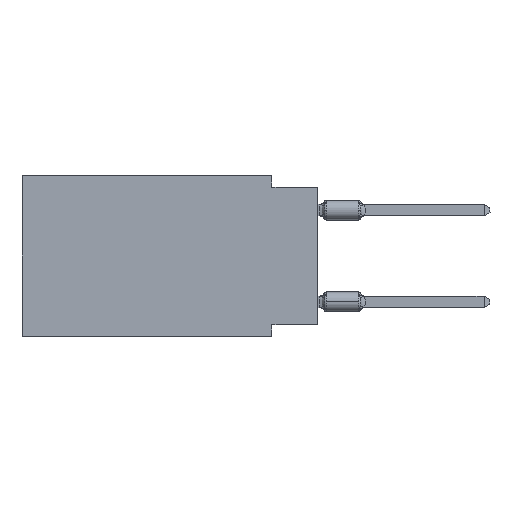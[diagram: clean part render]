
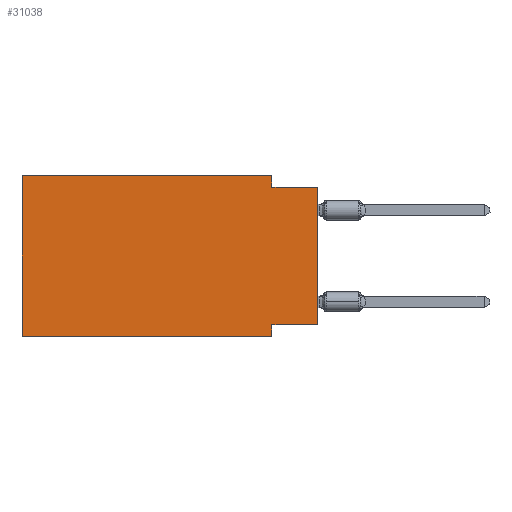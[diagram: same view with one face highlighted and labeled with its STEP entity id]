
A CAD part, left-side view. The second image highlights one B-rep face of the part: STEP entity #31038.
In plain terms, the highlighted planar face has unit normal (-1, 0, 0).
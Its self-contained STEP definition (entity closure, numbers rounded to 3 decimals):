
#113 = DIRECTION ( 'NONE',  ( 0., -1., 0. ) ) ;
#422 = VERTEX_POINT ( 'NONE', #11493 ) ;
#509 = DIRECTION ( 'NONE',  ( 0., 0., 1. ) ) ;
#956 = EDGE_CURVE ( 'NONE', #2455, #422, #2390, .T. ) ;
#1408 = EDGE_CURVE ( 'NONE', #10008, #23728, #19799, .T. ) ;
#2032 = VECTOR ( 'NONE', #21883, 1000. ) ;
#2119 = LINE ( 'NONE', #31627, #17342 ) ;
#2390 = LINE ( 'NONE', #9981, #16256 ) ;
#2455 = VERTEX_POINT ( 'NONE', #21975 ) ;
#3329 = VECTOR ( 'NONE', #509, 1000. ) ;
#3864 = VERTEX_POINT ( 'NONE', #25222 ) ;
#4171 = ORIENTED_EDGE ( 'NONE', *, *, #10172, .T. ) ;
#4334 = EDGE_CURVE ( 'NONE', #10008, #14365, #10883, .T. ) ;
#4459 = VECTOR ( 'NONE', #4576, 1000. ) ;
#4576 = DIRECTION ( 'NONE',  ( 0., -1., 0. ) ) ;
#5388 = ORIENTED_EDGE ( 'NONE', *, *, #7737, .F. ) ;
#5491 = CARTESIAN_POINT ( 'NONE',  ( 0., 16.383, -8.89 ) ) ;
#6189 = CARTESIAN_POINT ( 'NONE',  ( 0., 0., -8.255 ) ) ;
#6489 = DIRECTION ( 'NONE',  ( 0., -1., 0. ) ) ;
#7104 = FACE_OUTER_BOUND ( 'NONE', #15137, .T. ) ;
#7458 = DIRECTION ( 'NONE',  ( 0., 0., 1. ) ) ;
#7587 = DIRECTION ( 'NONE',  ( 0., 0., -1. ) ) ;
#7737 = EDGE_CURVE ( 'NONE', #7894, #2455, #2119, .T. ) ;
#7894 = VERTEX_POINT ( 'NONE', #5491 ) ;
#7901 = CARTESIAN_POINT ( 'NONE',  ( 0., 0., -0.635 ) ) ;
#8830 = LINE ( 'NONE', #15963, #19214 ) ;
#9702 = LINE ( 'NONE', #19440, #2032 ) ;
#9981 = CARTESIAN_POINT ( 'NONE',  ( 0., 16.383, 0. ) ) ;
#10008 = VERTEX_POINT ( 'NONE', #30984 ) ;
#10172 = EDGE_CURVE ( 'NONE', #7894, #23027, #18957, .T. ) ;
#10883 = LINE ( 'NONE', #6189, #26966 ) ;
#11108 = CARTESIAN_POINT ( 'NONE',  ( 0., 2.54, -8.89 ) ) ;
#11209 = DIRECTION ( 'NONE',  ( 0., 1., 0. ) ) ;
#11493 = CARTESIAN_POINT ( 'NONE',  ( 0., 2.54, 0. ) ) ;
#14095 = EDGE_CURVE ( 'NONE', #422, #3864, #9702, .T. ) ;
#14365 = VERTEX_POINT ( 'NONE', #18282 ) ;
#14409 = CARTESIAN_POINT ( 'NONE',  ( 0., 16.383, -8.89 ) ) ;
#15137 = EDGE_LOOP ( 'NONE', ( #27273, #29085, #23123, #18566, #5388, #4171, #16945, #26134 ) ) ;
#15963 = CARTESIAN_POINT ( 'NONE',  ( 0., 2.54, -8.89 ) ) ;
#16256 = VECTOR ( 'NONE', #113, 1000. ) ;
#16899 = VECTOR ( 'NONE', #6489, 1000. ) ;
#16945 = ORIENTED_EDGE ( 'NONE', *, *, #18250, .F. ) ;
#16979 = DIRECTION ( 'NONE',  ( 1., 0., 0. ) ) ;
#17342 = VECTOR ( 'NONE', #7458, 1000. ) ;
#18250 = EDGE_CURVE ( 'NONE', #14365, #23027, #8830, .T. ) ;
#18282 = CARTESIAN_POINT ( 'NONE',  ( 0., 2.54, -8.255 ) ) ;
#18566 = ORIENTED_EDGE ( 'NONE', *, *, #956, .F. ) ;
#18957 = LINE ( 'NONE', #14409, #16899 ) ;
#19214 = VECTOR ( 'NONE', #25850, 1000. ) ;
#19440 = CARTESIAN_POINT ( 'NONE',  ( 0., 2.54, 0. ) ) ;
#19799 = LINE ( 'NONE', #30021, #3329 ) ;
#21883 = DIRECTION ( 'NONE',  ( 0., 0., -1. ) ) ;
#21975 = CARTESIAN_POINT ( 'NONE',  ( 0., 16.383, 0. ) ) ;
#23027 = VERTEX_POINT ( 'NONE', #11108 ) ;
#23123 = ORIENTED_EDGE ( 'NONE', *, *, #14095, .F. ) ;
#23409 = AXIS2_PLACEMENT_3D ( 'NONE', #27194, #16979, #7587 ) ;
#23728 = VERTEX_POINT ( 'NONE', #7901 ) ;
#24502 = CARTESIAN_POINT ( 'NONE',  ( 0., 0., -0.635 ) ) ;
#24907 = EDGE_CURVE ( 'NONE', #3864, #23728, #29695, .T. ) ;
#25222 = CARTESIAN_POINT ( 'NONE',  ( 0., 2.54, -0.635 ) ) ;
#25850 = DIRECTION ( 'NONE',  ( 0., 0., -1. ) ) ;
#26134 = ORIENTED_EDGE ( 'NONE', *, *, #4334, .F. ) ;
#26966 = VECTOR ( 'NONE', #11209, 1000. ) ;
#27194 = CARTESIAN_POINT ( 'NONE',  ( 0., 16.383, 0. ) ) ;
#27273 = ORIENTED_EDGE ( 'NONE', *, *, #1408, .T. ) ;
#29085 = ORIENTED_EDGE ( 'NONE', *, *, #24907, .F. ) ;
#29313 = PLANE ( 'NONE',  #23409 ) ;
#29695 = LINE ( 'NONE', #24502, #4459 ) ;
#30021 = CARTESIAN_POINT ( 'NONE',  ( 0., 0., 0. ) ) ;
#30984 = CARTESIAN_POINT ( 'NONE',  ( 0., 0., -8.255 ) ) ;
#31038 = ADVANCED_FACE ( 'NONE', ( #7104 ), #29313, .F. ) ;
#31627 = CARTESIAN_POINT ( 'NONE',  ( 0., 16.383, 0. ) ) ;
